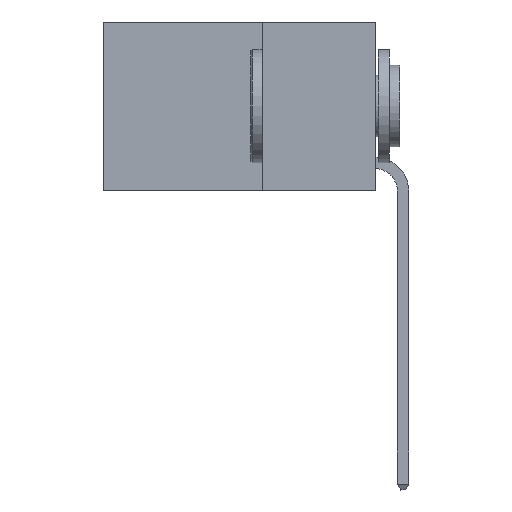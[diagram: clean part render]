
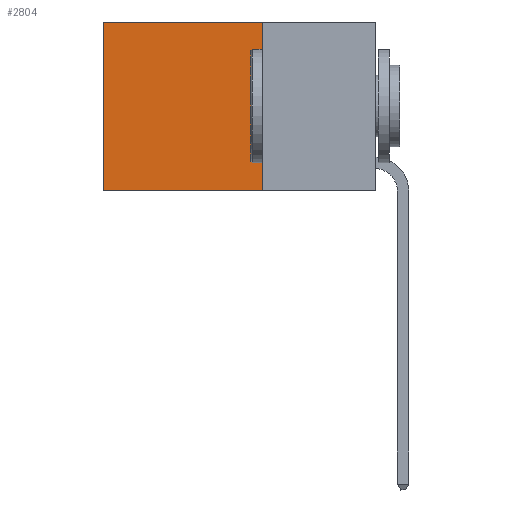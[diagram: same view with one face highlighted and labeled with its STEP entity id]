
A CAD part, left-side view. The second image highlights one B-rep face of the part: STEP entity #2804.
In plain terms, the highlighted planar face has unit normal (-1, 0, 0).
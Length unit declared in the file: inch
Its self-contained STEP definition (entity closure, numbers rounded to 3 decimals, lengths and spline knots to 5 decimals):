
#154 = DIRECTION ( 'NONE',  ( 0., 1., 0. ) ) ;
#330 = CARTESIAN_POINT ( 'NONE',  ( 0.2625, 0.25, -0.37 ) ) ;
#398 = DIRECTION ( 'NONE',  ( 0., 0., -1. ) ) ;
#408 = VERTEX_POINT ( 'NONE', #10493 ) ;
#503 = ORIENTED_EDGE ( 'NONE', *, *, #935, .T. ) ;
#835 = EDGE_CURVE ( 'NONE', #3286, #6195, #5941, .T. ) ;
#837 = VECTOR ( 'NONE', #154, 39.37008 ) ;
#935 = EDGE_CURVE ( 'NONE', #408, #9323, #8058, .T. ) ;
#2061 = CARTESIAN_POINT ( 'NONE',  ( 0.2625, 0.25, 0. ) ) ;
#2517 = CARTESIAN_POINT ( 'NONE',  ( 0.2625, 0.6, -0.37 ) ) ;
#2804 = ADVANCED_FACE ( 'NONE', ( #10505 ), #7092, .F. ) ;
#2934 = VECTOR ( 'NONE', #7848, 39.37008 ) ;
#2956 = DIRECTION ( 'NONE',  ( 1., 0., 0. ) ) ;
#3009 = CARTESIAN_POINT ( 'NONE',  ( 0.2625, 0.25, 0. ) ) ;
#3286 = VERTEX_POINT ( 'NONE', #330 ) ;
#3517 = LINE ( 'NONE', #7592, #6689 ) ;
#3822 = CARTESIAN_POINT ( 'NONE',  ( 0.2625, 0.6, 0. ) ) ;
#4065 = EDGE_CURVE ( 'NONE', #9323, #6195, #3517, .T. ) ;
#4349 = CARTESIAN_POINT ( 'NONE',  ( 0.2625, 0.25, -0.37 ) ) ;
#4674 = VECTOR ( 'NONE', #398, 39.37008 ) ;
#4697 = EDGE_LOOP ( 'NONE', ( #7004, #5083, #5930, #503 ) ) ;
#5083 = ORIENTED_EDGE ( 'NONE', *, *, #835, .F. ) ;
#5930 = ORIENTED_EDGE ( 'NONE', *, *, #8792, .F. ) ;
#5941 = LINE ( 'NONE', #4349, #837 ) ;
#6195 = VERTEX_POINT ( 'NONE', #2517 ) ;
#6542 = AXIS2_PLACEMENT_3D ( 'NONE', #3009, #2956, #9556 ) ;
#6689 = VECTOR ( 'NONE', #6778, 39.37008 ) ;
#6778 = DIRECTION ( 'NONE',  ( 0., 0., -1. ) ) ;
#7004 = ORIENTED_EDGE ( 'NONE', *, *, #4065, .T. ) ;
#7092 = PLANE ( 'NONE',  #6542 ) ;
#7592 = CARTESIAN_POINT ( 'NONE',  ( 0.2625, 0.6, 0. ) ) ;
#7848 = DIRECTION ( 'NONE',  ( 0., 1., 0. ) ) ;
#7936 = LINE ( 'NONE', #2061, #4674 ) ;
#8058 = LINE ( 'NONE', #9683, #2934 ) ;
#8792 = EDGE_CURVE ( 'NONE', #408, #3286, #7936, .T. ) ;
#9323 = VERTEX_POINT ( 'NONE', #3822 ) ;
#9556 = DIRECTION ( 'NONE',  ( 0., 0., -1. ) ) ;
#9683 = CARTESIAN_POINT ( 'NONE',  ( 0.2625, 0.25, 0. ) ) ;
#10493 = CARTESIAN_POINT ( 'NONE',  ( 0.2625, 0.25, 0. ) ) ;
#10505 = FACE_OUTER_BOUND ( 'NONE', #4697, .T. ) ;
